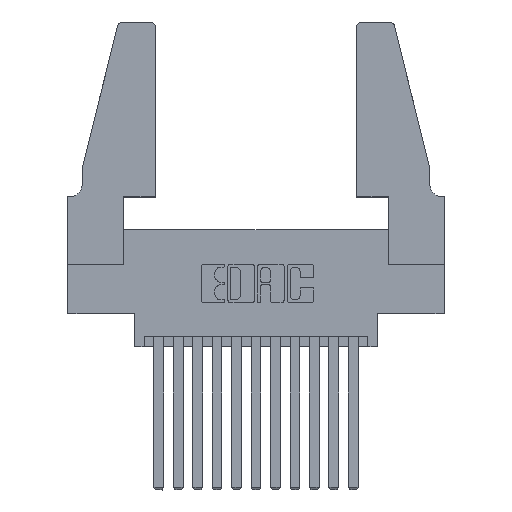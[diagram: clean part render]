
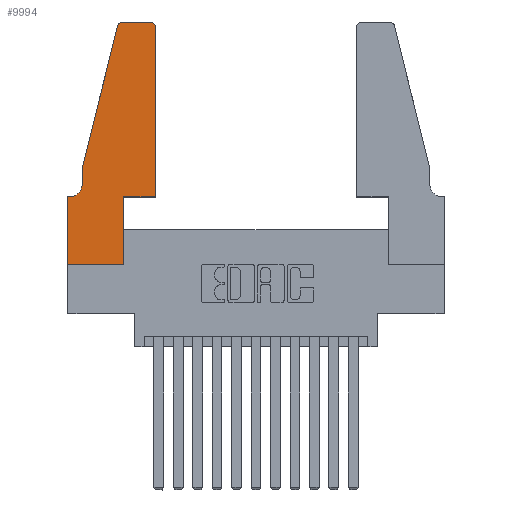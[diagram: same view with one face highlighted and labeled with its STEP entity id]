
A CAD part, top view. The second image highlights one B-rep face of the part: STEP entity #9994.
In plain terms, the highlighted planar face has unit normal (0, 0, 1).
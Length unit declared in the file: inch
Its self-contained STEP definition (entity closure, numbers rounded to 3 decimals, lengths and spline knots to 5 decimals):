
#313 = VERTEX_POINT ( 'NONE', #5158 ) ;
#777 = CARTESIAN_POINT ( 'NONE',  ( 0.0755, 0.35, 0.37 ) ) ;
#1022 = CARTESIAN_POINT ( 'NONE',  ( 0.284, 1.22, 0.37 ) ) ;
#1135 = FACE_OUTER_BOUND ( 'NONE', #3489, .T. ) ;
#1506 = CARTESIAN_POINT ( 'NONE',  ( 0.4505, 1.22, 0.37 ) ) ;
#1687 = EDGE_CURVE ( 'NONE', #5415, #9586, #12926, .T. ) ;
#1689 = LINE ( 'NONE', #2347, #9051 ) ;
#1700 = VERTEX_POINT ( 'NONE', #2002 ) ;
#1894 = AXIS2_PLACEMENT_3D ( 'NONE', #4901, #14043, #12845 ) ;
#1997 = LINE ( 'NONE', #4690, #4335 ) ;
#2002 = CARTESIAN_POINT ( 'NONE',  ( 0.4505, 0.35, 0.37 ) ) ;
#2288 = EDGE_CURVE ( 'NONE', #13725, #4343, #8599, .T. ) ;
#2347 = CARTESIAN_POINT ( 'NONE',  ( 0.4505, 0.35, 0.37 ) ) ;
#2440 = CARTESIAN_POINT ( 'NONE',  ( 0.0755, 0.42, 0.37 ) ) ;
#2940 = DIRECTION ( 'NONE',  ( -1., 0., 0. ) ) ;
#2964 = VECTOR ( 'NONE', #6287, 39.37008 ) ;
#3143 = DIRECTION ( 'NONE',  ( 0., 0., 1. ) ) ;
#3177 = LINE ( 'NONE', #5696, #5528 ) ;
#3283 = DIRECTION ( 'NONE',  ( 1., 0., 0. ) ) ;
#3446 = LINE ( 'NONE', #13032, #3985 ) ;
#3489 = EDGE_LOOP ( 'NONE', ( #3759, #6807, #10052, #6531, #12851, #7740, #13252, #12808, #14656, #6244, #9009, #8389 ) ) ;
#3492 = AXIS2_PLACEMENT_3D ( 'NONE', #8138, #11397, #8082 ) ;
#3544 = CARTESIAN_POINT ( 'NONE',  ( 0.0755, 0.5, 0.37 ) ) ;
#3582 = VERTEX_POINT ( 'NONE', #3544 ) ;
#3759 = ORIENTED_EDGE ( 'NONE', *, *, #10833, .T. ) ;
#3874 = EDGE_CURVE ( 'NONE', #9948, #7113, #10146, .T. ) ;
#3985 = VECTOR ( 'NONE', #13140, 39.37008 ) ;
#3993 = LINE ( 'NONE', #11935, #4191 ) ;
#4191 = VECTOR ( 'NONE', #14385, 39.37008 ) ;
#4282 = LINE ( 'NONE', #777, #10032 ) ;
#4335 = VECTOR ( 'NONE', #9216, 39.37008 ) ;
#4343 = VERTEX_POINT ( 'NONE', #13114 ) ;
#4690 = CARTESIAN_POINT ( 'NONE',  ( 0., 0., 0.37 ) ) ;
#4719 = VERTEX_POINT ( 'NONE', #14474 ) ;
#4760 = VERTEX_POINT ( 'NONE', #13280 ) ;
#4822 = CARTESIAN_POINT ( 'NONE',  ( 0.0755, 0.5, 0.37 ) ) ;
#4901 = CARTESIAN_POINT ( 'NONE',  ( 0.4205, 1.22, 0.37 ) ) ;
#4945 = LINE ( 'NONE', #4822, #10144 ) ;
#5080 = EDGE_CURVE ( 'NONE', #1700, #13725, #1689, .T. ) ;
#5158 = CARTESIAN_POINT ( 'NONE',  ( 0., 0., 0.37 ) ) ;
#5208 = VERTEX_POINT ( 'NONE', #2440 ) ;
#5278 = CARTESIAN_POINT ( 'NONE',  ( 0.2865, 0.35, 0.37 ) ) ;
#5413 = EDGE_CURVE ( 'NONE', #4760, #4719, #4282, .T. ) ;
#5415 = VERTEX_POINT ( 'NONE', #11072 ) ;
#5528 = VECTOR ( 'NONE', #12601, 39.37008 ) ;
#5630 = EDGE_CURVE ( 'NONE', #313, #9948, #1997, .T. ) ;
#5696 = CARTESIAN_POINT ( 'NONE',  ( 0.4505, 0.35, 0.37 ) ) ;
#5717 = CIRCLE ( 'NONE', #9450, 0.07 ) ;
#6244 = ORIENTED_EDGE ( 'NONE', *, *, #8051, .T. ) ;
#6285 = CARTESIAN_POINT ( 'NONE',  ( 0., 0., 0.37 ) ) ;
#6287 = DIRECTION ( 'NONE',  ( 0., 1., 0. ) ) ;
#6531 = ORIENTED_EDGE ( 'NONE', *, *, #13800, .T. ) ;
#6807 = ORIENTED_EDGE ( 'NONE', *, *, #1687, .T. ) ;
#6873 = CARTESIAN_POINT ( 'NONE',  ( 0.0055, 0.42, 0.37 ) ) ;
#7113 = VERTEX_POINT ( 'NONE', #5278 ) ;
#7621 = CARTESIAN_POINT ( 'NONE',  ( 0.2865, 0.35, 0.37 ) ) ;
#7740 = ORIENTED_EDGE ( 'NONE', *, *, #5413, .T. ) ;
#8051 = EDGE_CURVE ( 'NONE', #7113, #1700, #3177, .T. ) ;
#8082 = DIRECTION ( 'NONE',  ( 1., 0., 0. ) ) ;
#8137 = EDGE_CURVE ( 'NONE', #5208, #4760, #5717, .T. ) ;
#8138 = CARTESIAN_POINT ( 'NONE',  ( 0., 0.35, 0.37 ) ) ;
#8389 = ORIENTED_EDGE ( 'NONE', *, *, #2288, .T. ) ;
#8599 = CIRCLE ( 'NONE', #1894, 0.03 ) ;
#8724 = VECTOR ( 'NONE', #14364, 39.37008 ) ;
#9009 = ORIENTED_EDGE ( 'NONE', *, *, #5080, .T. ) ;
#9051 = VECTOR ( 'NONE', #11637, 39.37008 ) ;
#9055 = DIRECTION ( 'NONE',  ( -1., 0., 0. ) ) ;
#9216 = DIRECTION ( 'NONE',  ( 1., 0., 0. ) ) ;
#9450 = AXIS2_PLACEMENT_3D ( 'NONE', #6873, #10319, #9055 ) ;
#9555 = EDGE_CURVE ( 'NONE', #9586, #3582, #4945, .T. ) ;
#9586 = VERTEX_POINT ( 'NONE', #9801 ) ;
#9686 = EDGE_CURVE ( 'NONE', #4719, #313, #11227, .T. ) ;
#9801 = CARTESIAN_POINT ( 'NONE',  ( 0.25487, 1.22718, 0.37 ) ) ;
#9948 = VERTEX_POINT ( 'NONE', #13728 ) ;
#9994 = ADVANCED_FACE ( 'NONE', ( #1135 ), #10285, .T. ) ;
#10032 = VECTOR ( 'NONE', #2940, 39.37008 ) ;
#10052 = ORIENTED_EDGE ( 'NONE', *, *, #9555, .T. ) ;
#10144 = VECTOR ( 'NONE', #14106, 39.37008 ) ;
#10146 = LINE ( 'NONE', #7621, #2964 ) ;
#10285 = PLANE ( 'NONE',  #3492 ) ;
#10319 = DIRECTION ( 'NONE',  ( 0., 0., -1. ) ) ;
#10833 = EDGE_CURVE ( 'NONE', #4343, #5415, #3993, .T. ) ;
#11072 = CARTESIAN_POINT ( 'NONE',  ( 0.284, 1.25, 0.37 ) ) ;
#11227 = LINE ( 'NONE', #6285, #8724 ) ;
#11397 = DIRECTION ( 'NONE',  ( 0., 0., 1. ) ) ;
#11637 = DIRECTION ( 'NONE',  ( 0., 1., 0. ) ) ;
#11935 = CARTESIAN_POINT ( 'NONE',  ( 0.2605, 1.25, 0.37 ) ) ;
#12601 = DIRECTION ( 'NONE',  ( 1., 0., 0. ) ) ;
#12808 = ORIENTED_EDGE ( 'NONE', *, *, #5630, .T. ) ;
#12845 = DIRECTION ( 'NONE',  ( 1., 0., 0. ) ) ;
#12851 = ORIENTED_EDGE ( 'NONE', *, *, #8137, .T. ) ;
#12926 = CIRCLE ( 'NONE', #14267, 0.03 ) ;
#13032 = CARTESIAN_POINT ( 'NONE',  ( 0.0755, 0.5, 0.37 ) ) ;
#13114 = CARTESIAN_POINT ( 'NONE',  ( 0.4205, 1.25, 0.37 ) ) ;
#13140 = DIRECTION ( 'NONE',  ( 0., -1., 0. ) ) ;
#13252 = ORIENTED_EDGE ( 'NONE', *, *, #9686, .T. ) ;
#13280 = CARTESIAN_POINT ( 'NONE',  ( 0.0055, 0.35, 0.37 ) ) ;
#13725 = VERTEX_POINT ( 'NONE', #1506 ) ;
#13728 = CARTESIAN_POINT ( 'NONE',  ( 0.2865, 0., 0.37 ) ) ;
#13800 = EDGE_CURVE ( 'NONE', #3582, #5208, #3446, .T. ) ;
#14043 = DIRECTION ( 'NONE',  ( 0., 0., 1. ) ) ;
#14106 = DIRECTION ( 'NONE',  ( -0.239, -0.971, 0. ) ) ;
#14267 = AXIS2_PLACEMENT_3D ( 'NONE', #1022, #3143, #3283 ) ;
#14364 = DIRECTION ( 'NONE',  ( 0., -1., 0. ) ) ;
#14385 = DIRECTION ( 'NONE',  ( -1., 0., 0. ) ) ;
#14474 = CARTESIAN_POINT ( 'NONE',  ( 0., 0.35, 0.37 ) ) ;
#14656 = ORIENTED_EDGE ( 'NONE', *, *, #3874, .T. ) ;
